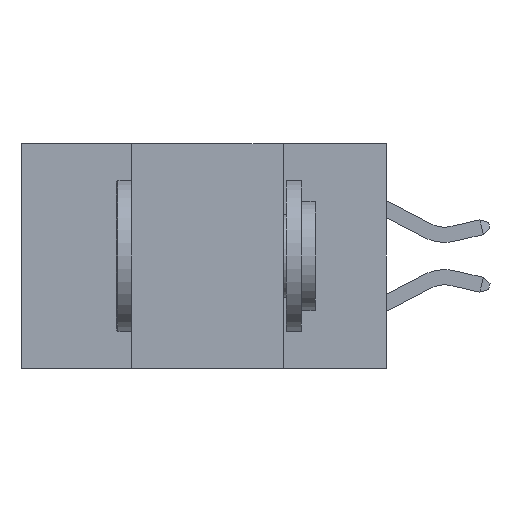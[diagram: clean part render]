
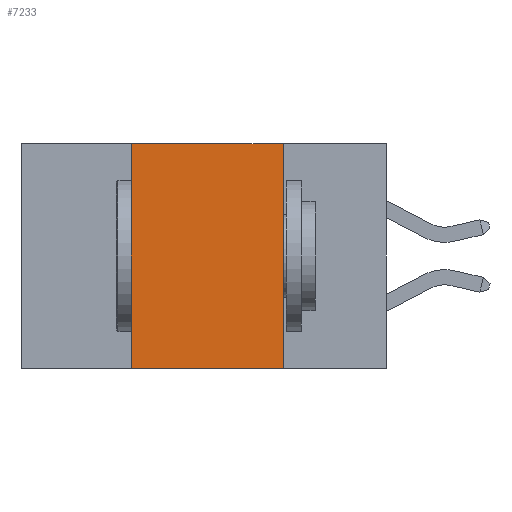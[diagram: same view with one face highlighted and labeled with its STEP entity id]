
A CAD part, left-side view. The second image highlights one B-rep face of the part: STEP entity #7233.
In plain terms, the highlighted planar face has unit normal (-1, 0, 0).
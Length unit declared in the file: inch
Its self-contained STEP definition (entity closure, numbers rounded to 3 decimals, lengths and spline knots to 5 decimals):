
#13 = EDGE_CURVE ( 'NONE', #3582, #3821, #8240, .T. ) ;
#486 = EDGE_LOOP ( 'NONE', ( #5145, #7258, #913, #3183 ) ) ;
#586 = CARTESIAN_POINT ( 'NONE',  ( 0., 0.6, -0.37 ) ) ;
#913 = ORIENTED_EDGE ( 'NONE', *, *, #13, .F. ) ;
#1191 = VERTEX_POINT ( 'NONE', #5148 ) ;
#1632 = CARTESIAN_POINT ( 'NONE',  ( 0., 0.42, -0.37 ) ) ;
#1726 = EDGE_CURVE ( 'NONE', #3821, #1191, #3378, .T. ) ;
#2283 = PLANE ( 'NONE',  #5068 ) ;
#2321 = EDGE_CURVE ( 'NONE', #1191, #4668, #3057, .T. ) ;
#2338 = DIRECTION ( 'NONE',  ( 0., -1., 0. ) ) ;
#3057 = LINE ( 'NONE', #8215, #9263 ) ;
#3101 = CARTESIAN_POINT ( 'NONE',  ( 0., 0.6, 0. ) ) ;
#3145 = VECTOR ( 'NONE', #2338, 39.37008 ) ;
#3183 = ORIENTED_EDGE ( 'NONE', *, *, #10102, .T. ) ;
#3378 = LINE ( 'NONE', #5168, #5561 ) ;
#3582 = VERTEX_POINT ( 'NONE', #9556 ) ;
#3821 = VERTEX_POINT ( 'NONE', #8163 ) ;
#3969 = DIRECTION ( 'NONE',  ( 0., 0., -1. ) ) ;
#4073 = CARTESIAN_POINT ( 'NONE',  ( 0., 0.17, -0.37 ) ) ;
#4668 = VERTEX_POINT ( 'NONE', #4073 ) ;
#5068 = AXIS2_PLACEMENT_3D ( 'NONE', #3101, #8769, #3969 ) ;
#5145 = ORIENTED_EDGE ( 'NONE', *, *, #2321, .F. ) ;
#5148 = CARTESIAN_POINT ( 'NONE',  ( 0., 0.17, 0. ) ) ;
#5168 = CARTESIAN_POINT ( 'NONE',  ( 0., 0.6, 0. ) ) ;
#5201 = DIRECTION ( 'NONE',  ( 0., -1., 0. ) ) ;
#5561 = VECTOR ( 'NONE', #5201, 39.37008 ) ;
#5833 = VECTOR ( 'NONE', #8681, 39.37008 ) ;
#5869 = DIRECTION ( 'NONE',  ( 0., 0., -1. ) ) ;
#6665 = FACE_OUTER_BOUND ( 'NONE', #486, .T. ) ;
#7233 = ADVANCED_FACE ( 'NONE', ( #6665 ), #2283, .F. ) ;
#7258 = ORIENTED_EDGE ( 'NONE', *, *, #1726, .F. ) ;
#7484 = LINE ( 'NONE', #586, #3145 ) ;
#8163 = CARTESIAN_POINT ( 'NONE',  ( 0., 0.42, 0. ) ) ;
#8215 = CARTESIAN_POINT ( 'NONE',  ( 0., 0.17, -0.37 ) ) ;
#8240 = LINE ( 'NONE', #1632, #5833 ) ;
#8681 = DIRECTION ( 'NONE',  ( 0., 0., 1. ) ) ;
#8769 = DIRECTION ( 'NONE',  ( 1., 0., 0. ) ) ;
#9263 = VECTOR ( 'NONE', #5869, 39.37008 ) ;
#9556 = CARTESIAN_POINT ( 'NONE',  ( 0., 0.42, -0.37 ) ) ;
#10102 = EDGE_CURVE ( 'NONE', #3582, #4668, #7484, .T. ) ;
